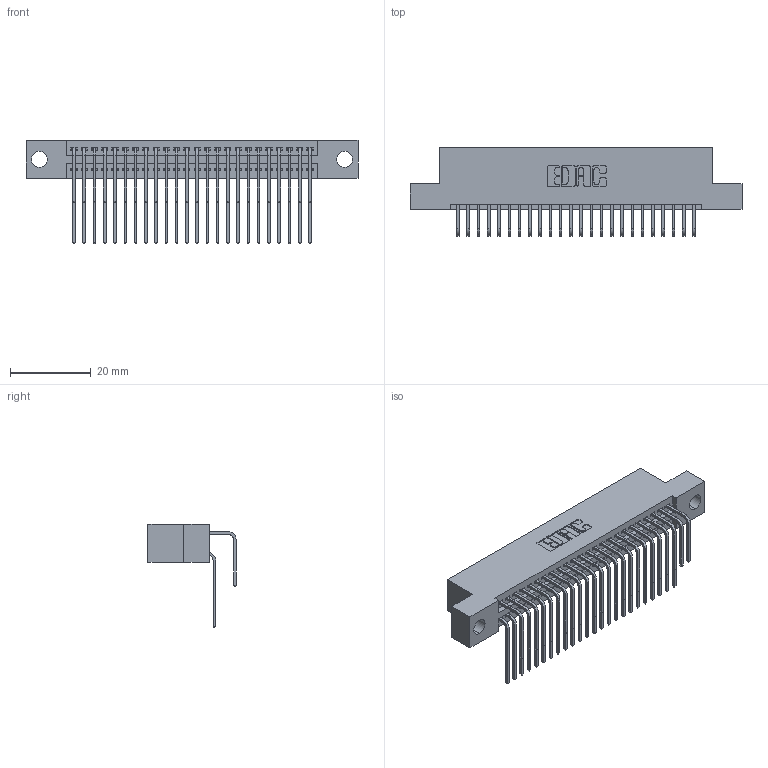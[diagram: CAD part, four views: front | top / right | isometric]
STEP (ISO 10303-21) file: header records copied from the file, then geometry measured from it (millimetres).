
FILE_DESCRIPTION (( 'STEP AP203' ), '1' );
FILE_NAME ('395-048-558-204.STEP', '2021-06-16T23:37:09', ( '' ), ( '' ), 'SwSTEP 2.0', 'SolidWorks 2020', '' );
FILE_SCHEMA (( 'CONFIG_CONTROL_DESIGN' ));
Length unit declared in the file: inch
Products named in the file (4): 395-048-558-204; 345 Part_Flush Mounting Lugs - 0.156 Dia-TI; 345-292-001_558 Tail - 2; 345-292-001_558 559 Tail - 1
Assembly tree (49 placements, depth 2):
  395-048-558-204
    345 Part_Flush Mounting Lugs - 0.156 Dia-TI
    345-292-001_558 559 Tail - 1  x24
    345-292-001_558 Tail - 2  x24
Bounding box: 82.17 x 21.83 x 25.53 mm (x, y, z)
Volume: 7985.8 mm3; surface area: 12609.5 mm2
Topology: 49 solids, 49 shells, 2636 faces, 7817 edges, 5146 vertices
Faces by surface type: plane 1774, cylinder 862
Entity records: 23325 total; most frequent: CARTESIAN_POINT 3977, ORIENTED_EDGE 3858, DIRECTION 3501, EDGE_CURVE 1929, VECTOR 1661, LINE 1661, VERTEX_POINT 1282, AXIS2_PLACEMENT_3D 920
